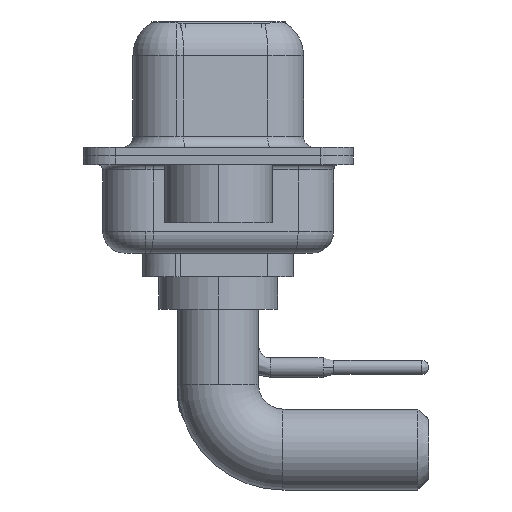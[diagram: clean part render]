
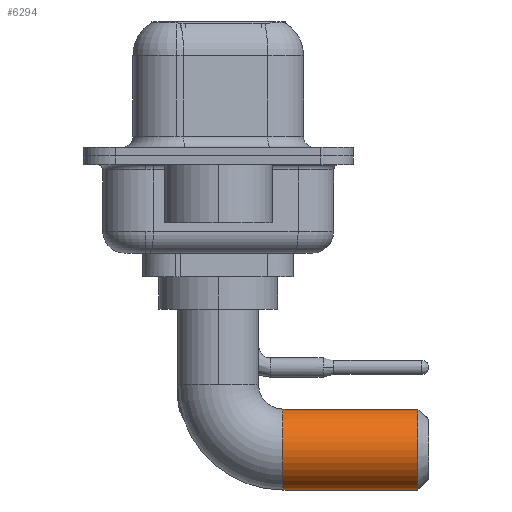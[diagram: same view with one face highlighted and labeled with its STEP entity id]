
A CAD part, left-side view. The second image highlights one B-rep face of the part: STEP entity #6294.
In plain terms, the highlighted cylindrical face has radius 1.875 mm (diameter 3.75 mm), a partial arc.
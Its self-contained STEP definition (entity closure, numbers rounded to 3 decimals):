
#297 = ORIENTED_EDGE ( 'NONE', *, *, #17077, .T. ) ;
#312 = EDGE_CURVE ( 'NONE', #14141, #16417, #22297, .T. ) ;
#379 = AXIS2_PLACEMENT_3D ( 'NONE', #20830, #11284, #7910 ) ;
#1488 = CARTESIAN_POINT ( 'NONE',  ( 0., -9.25, -4.625 ) ) ;
#2172 = DIRECTION ( 'NONE',  ( 0., -1., 0. ) ) ;
#2176 = CARTESIAN_POINT ( 'NONE',  ( 0., -3., -8.375 ) ) ;
#2530 = DIRECTION ( 'NONE',  ( 0., -1., 0. ) ) ;
#2707 = DIRECTION ( 'NONE',  ( -1., 0., 0. ) ) ;
#3048 = AXIS2_PLACEMENT_3D ( 'NONE', #6011, #2172, #13251 ) ;
#3818 = ORIENTED_EDGE ( 'NONE', *, *, #21887, .T. ) ;
#5898 = CYLINDRICAL_SURFACE ( 'NONE', #3048, 1.875 ) ;
#6011 = CARTESIAN_POINT ( 'NONE',  ( 0., -3., -6.5 ) ) ;
#6294 = ADVANCED_FACE ( 'NONE', ( #9869 ), #5898, .T. ) ;
#6621 = CARTESIAN_POINT ( 'NONE',  ( 0., -9.25, -8.375 ) ) ;
#7198 = ORIENTED_EDGE ( 'NONE', *, *, #312, .F. ) ;
#7458 = DIRECTION ( 'NONE',  ( 0., -1., 0. ) ) ;
#7910 = DIRECTION ( 'NONE',  ( 0., 0., -1. ) ) ;
#8277 = CARTESIAN_POINT ( 'NONE',  ( 0., -3., -6.5 ) ) ;
#9832 = DIRECTION ( 'NONE',  ( 0., -1., 0. ) ) ;
#9869 = FACE_OUTER_BOUND ( 'NONE', #17440, .T. ) ;
#11284 = DIRECTION ( 'NONE',  ( 0., 1., 0. ) ) ;
#12398 = VERTEX_POINT ( 'NONE', #14811 ) ;
#12659 = CARTESIAN_POINT ( 'NONE',  ( 0., -3., -4.625 ) ) ;
#13251 = DIRECTION ( 'NONE',  ( 0., 0., -1. ) ) ;
#13758 = VECTOR ( 'NONE', #2530, 1000. ) ;
#14141 = VERTEX_POINT ( 'NONE', #12659 ) ;
#14811 = CARTESIAN_POINT ( 'NONE',  ( 0., -3., -8.375 ) ) ;
#14843 = EDGE_CURVE ( 'NONE', #14141, #12398, #17927, .T. ) ;
#16164 = VERTEX_POINT ( 'NONE', #6621 ) ;
#16417 = VERTEX_POINT ( 'NONE', #1488 ) ;
#16557 = CIRCLE ( 'NONE', #379, 1.875 ) ;
#16740 = CARTESIAN_POINT ( 'NONE',  ( 0., -3., -4.625 ) ) ;
#17077 = EDGE_CURVE ( 'NONE', #12398, #16164, #22808, .T. ) ;
#17440 = EDGE_LOOP ( 'NONE', ( #7198, #21878, #297, #3818 ) ) ;
#17927 = CIRCLE ( 'NONE', #20652, 1.875 ) ;
#18434 = VECTOR ( 'NONE', #7458, 1000. ) ;
#20652 = AXIS2_PLACEMENT_3D ( 'NONE', #8277, #9832, #2707 ) ;
#20830 = CARTESIAN_POINT ( 'NONE',  ( 0., -9.25, -6.5 ) ) ;
#21878 = ORIENTED_EDGE ( 'NONE', *, *, #14843, .T. ) ;
#21887 = EDGE_CURVE ( 'NONE', #16164, #16417, #16557, .T. ) ;
#22297 = LINE ( 'NONE', #16740, #18434 ) ;
#22808 = LINE ( 'NONE', #2176, #13758 ) ;
